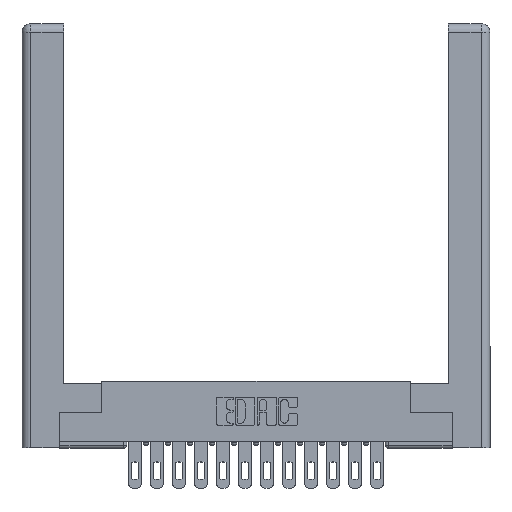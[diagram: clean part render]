
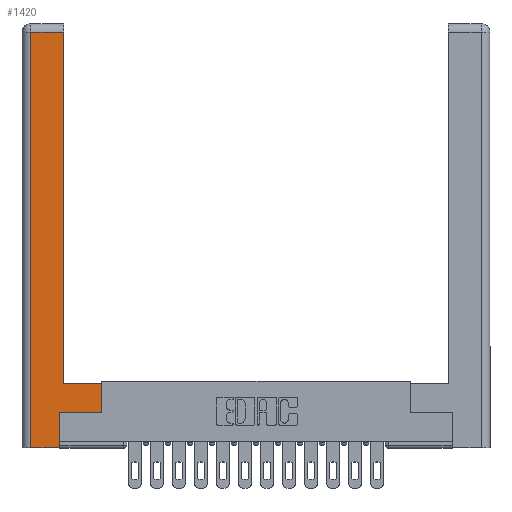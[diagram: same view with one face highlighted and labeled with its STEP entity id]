
A CAD part, top view. The second image highlights one B-rep face of the part: STEP entity #1420.
In plain terms, the highlighted planar face has unit normal (0, 0, 1).
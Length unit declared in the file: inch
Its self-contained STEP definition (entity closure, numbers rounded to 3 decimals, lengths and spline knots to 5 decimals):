
#4 = VECTOR ( 'NONE', #12552, 39.37008 ) ;
#13 = CARTESIAN_POINT ( 'NONE',  ( 0., 0., 0. ) ) ;
#21 = LINE ( 'NONE', #12052, #10022 ) ;
#232 = CARTESIAN_POINT ( 'NONE',  ( 0.265, 0.245, 0. ) ) ;
#280 = DIRECTION ( 'NONE',  ( -1., 0., 0. ) ) ;
#433 = DIRECTION ( 'NONE',  ( 0., 1., 0. ) ) ;
#507 = CARTESIAN_POINT ( 'NONE',  ( 0.295, 3., 0. ) ) ;
#829 = VECTOR ( 'NONE', #2797, 39.37008 ) ;
#1042 = VERTEX_POINT ( 'NONE', #15415 ) ;
#1375 = ORIENTED_EDGE ( 'NONE', *, *, #2324, .T. ) ;
#1420 = ADVANCED_FACE ( 'NONE', ( #15540 ), #10288, .F. ) ;
#1540 = VECTOR ( 'NONE', #10616, 39.37008 ) ;
#1595 = VERTEX_POINT ( 'NONE', #14770 ) ;
#2324 = EDGE_CURVE ( 'NONE', #16611, #1042, #10836, .T. ) ;
#2726 = CARTESIAN_POINT ( 'NONE',  ( 0.565, 0.45, 0. ) ) ;
#2744 = CARTESIAN_POINT ( 'NONE',  ( 0.0615, 0., 0. ) ) ;
#2797 = DIRECTION ( 'NONE',  ( 0., 1., 0. ) ) ;
#3009 = ORIENTED_EDGE ( 'NONE', *, *, #10083, .T. ) ;
#3119 = CARTESIAN_POINT ( 'NONE',  ( 0.565, 0.245, 0. ) ) ;
#4198 = ORIENTED_EDGE ( 'NONE', *, *, #16479, .T. ) ;
#4206 = CARTESIAN_POINT ( 'NONE',  ( 0.0615, 2.94, 0. ) ) ;
#4307 = VERTEX_POINT ( 'NONE', #9776 ) ;
#4998 = LINE ( 'NONE', #14461, #1540 ) ;
#5037 = ORIENTED_EDGE ( 'NONE', *, *, #12401, .T. ) ;
#5446 = CARTESIAN_POINT ( 'NONE',  ( 0.295, 2.94, 0. ) ) ;
#5666 = VERTEX_POINT ( 'NONE', #2744 ) ;
#5845 = VECTOR ( 'NONE', #9331, 39.37008 ) ;
#6545 = VERTEX_POINT ( 'NONE', #8633 ) ;
#6696 = LINE ( 'NONE', #7795, #5845 ) ;
#7115 = ORIENTED_EDGE ( 'NONE', *, *, #13950, .T. ) ;
#7345 = VECTOR ( 'NONE', #280, 39.37008 ) ;
#7504 = LINE ( 'NONE', #15829, #14064 ) ;
#7555 = ORIENTED_EDGE ( 'NONE', *, *, #14593, .T. ) ;
#7795 = CARTESIAN_POINT ( 'NONE',  ( 0.0615, 0., 0. ) ) ;
#8390 = VECTOR ( 'NONE', #433, 39.37008 ) ;
#8633 = CARTESIAN_POINT ( 'NONE',  ( 0.265, 0., 0. ) ) ;
#9270 = DIRECTION ( 'NONE',  ( -1., 0., 0. ) ) ;
#9331 = DIRECTION ( 'NONE',  ( 0., -1., 0. ) ) ;
#9776 = CARTESIAN_POINT ( 'NONE',  ( 0.565, 0.45, 0. ) ) ;
#10022 = VECTOR ( 'NONE', #10730, 39.37008 ) ;
#10083 = EDGE_CURVE ( 'NONE', #14329, #11828, #21, .T. ) ;
#10084 = CARTESIAN_POINT ( 'NONE',  ( 0.265, 0.245, 0. ) ) ;
#10119 = EDGE_CURVE ( 'NONE', #6545, #14329, #12469, .T. ) ;
#10288 = PLANE ( 'NONE',  #11927 ) ;
#10328 = EDGE_CURVE ( 'NONE', #1595, #16611, #15581, .T. ) ;
#10616 = DIRECTION ( 'NONE',  ( 1., 0., 0. ) ) ;
#10730 = DIRECTION ( 'NONE',  ( 1., 0., 0. ) ) ;
#10836 = LINE ( 'NONE', #4206, #7345 ) ;
#11195 = EDGE_LOOP ( 'NONE', ( #11425, #1375, #4198, #7115, #13165, #3009, #7555, #5037 ) ) ;
#11425 = ORIENTED_EDGE ( 'NONE', *, *, #10328, .T. ) ;
#11828 = VERTEX_POINT ( 'NONE', #3119 ) ;
#11927 = AXIS2_PLACEMENT_3D ( 'NONE', #13, #12936, #14309 ) ;
#12052 = CARTESIAN_POINT ( 'NONE',  ( 0.565, 0.245, 0. ) ) ;
#12401 = EDGE_CURVE ( 'NONE', #4307, #1595, #7504, .T. ) ;
#12469 = LINE ( 'NONE', #232, #829 ) ;
#12552 = DIRECTION ( 'NONE',  ( 0., 1., 0. ) ) ;
#12936 = DIRECTION ( 'NONE',  ( 0., 0., -1. ) ) ;
#13165 = ORIENTED_EDGE ( 'NONE', *, *, #10119, .T. ) ;
#13950 = EDGE_CURVE ( 'NONE', #5666, #6545, #4998, .T. ) ;
#14064 = VECTOR ( 'NONE', #9270, 39.37008 ) ;
#14309 = DIRECTION ( 'NONE',  ( -1., 0., 0. ) ) ;
#14329 = VERTEX_POINT ( 'NONE', #10084 ) ;
#14461 = CARTESIAN_POINT ( 'NONE',  ( 0.265, 0., 0. ) ) ;
#14583 = LINE ( 'NONE', #2726, #8390 ) ;
#14593 = EDGE_CURVE ( 'NONE', #11828, #4307, #14583, .T. ) ;
#14770 = CARTESIAN_POINT ( 'NONE',  ( 0.295, 0.45, 0. ) ) ;
#15415 = CARTESIAN_POINT ( 'NONE',  ( 0.0615, 2.94, 0. ) ) ;
#15540 = FACE_OUTER_BOUND ( 'NONE', #11195, .T. ) ;
#15581 = LINE ( 'NONE', #507, #4 ) ;
#15829 = CARTESIAN_POINT ( 'NONE',  ( 0.295, 0.45, 0. ) ) ;
#16479 = EDGE_CURVE ( 'NONE', #1042, #5666, #6696, .T. ) ;
#16611 = VERTEX_POINT ( 'NONE', #5446 ) ;
